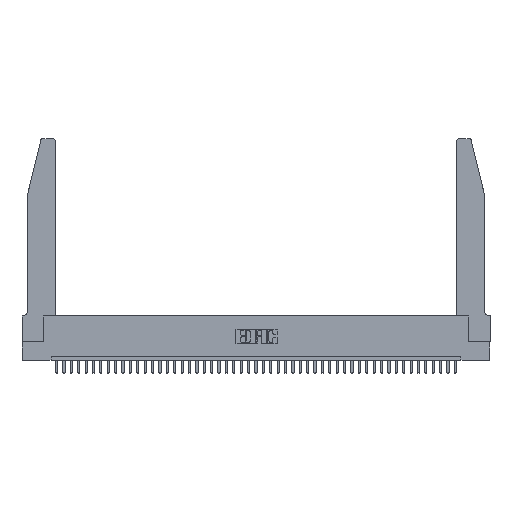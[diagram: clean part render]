
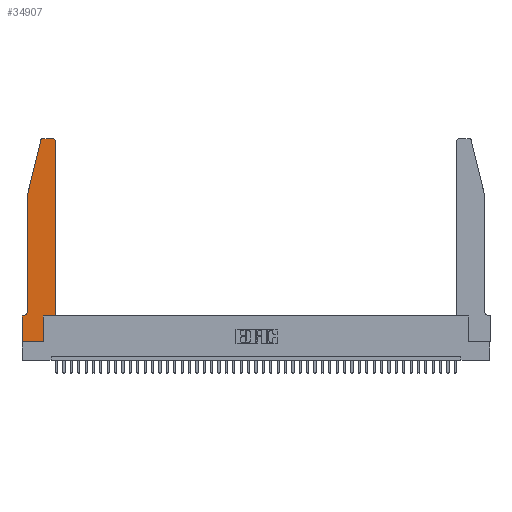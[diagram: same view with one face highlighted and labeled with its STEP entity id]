
A CAD part, top view. The second image highlights one B-rep face of the part: STEP entity #34907.
In plain terms, the highlighted planar face has unit normal (0, 0, 1).
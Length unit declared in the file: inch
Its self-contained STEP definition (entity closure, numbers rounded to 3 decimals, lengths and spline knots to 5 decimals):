
#297 = DIRECTION ( 'NONE',  ( 1., 0., 0. ) ) ;
#403 = CARTESIAN_POINT ( 'NONE',  ( 0., 0.35, 0.37 ) ) ;
#1978 = EDGE_CURVE ( 'NONE', #20768, #39292, #31162, .T. ) ;
#2014 = DIRECTION ( 'NONE',  ( -0.239, -0.971, 0. ) ) ;
#2106 = ORIENTED_EDGE ( 'NONE', *, *, #39608, .T. ) ;
#2796 = LINE ( 'NONE', #20303, #14570 ) ;
#3022 = EDGE_CURVE ( 'NONE', #9658, #12746, #7732, .T. ) ;
#3857 = EDGE_CURVE ( 'NONE', #33900, #9658, #42615, .T. ) ;
#4314 = EDGE_CURVE ( 'NONE', #7979, #17851, #2796, .T. ) ;
#4957 = CARTESIAN_POINT ( 'NONE',  ( 0.284, 2.75, 0.37 ) ) ;
#5956 = AXIS2_PLACEMENT_3D ( 'NONE', #39282, #18823, #28895 ) ;
#6140 = DIRECTION ( 'NONE',  ( 1., 0., 0. ) ) ;
#6645 = VECTOR ( 'NONE', #2014, 39.37008 ) ;
#6658 = DIRECTION ( 'NONE',  ( 0., 1., 0. ) ) ;
#6995 = CARTESIAN_POINT ( 'NONE',  ( 0.4505, 0.35, 0.37 ) ) ;
#7254 = VERTEX_POINT ( 'NONE', #19787 ) ;
#7298 = PLANE ( 'NONE',  #24226 ) ;
#7732 = LINE ( 'NONE', #34186, #6645 ) ;
#7979 = VERTEX_POINT ( 'NONE', #23984 ) ;
#8197 = ORIENTED_EDGE ( 'NONE', *, *, #4314, .T. ) ;
#9658 = VERTEX_POINT ( 'NONE', #10360 ) ;
#9827 = DIRECTION ( 'NONE',  ( 0., 0., 1. ) ) ;
#10360 = CARTESIAN_POINT ( 'NONE',  ( 0.25487, 2.72718, 0.37 ) ) ;
#10837 = CARTESIAN_POINT ( 'NONE',  ( 0.0755, 2., 0.37 ) ) ;
#10908 = DIRECTION ( 'NONE',  ( 1., 0., 0. ) ) ;
#11545 = CARTESIAN_POINT ( 'NONE',  ( 0.2865, 0.35, 0.37 ) ) ;
#11945 = CARTESIAN_POINT ( 'NONE',  ( 0.4505, 0.35, 0.37 ) ) ;
#12109 = DIRECTION ( 'NONE',  ( 0., 1., 0. ) ) ;
#12197 = CARTESIAN_POINT ( 'NONE',  ( 0., 0., 0.37 ) ) ;
#12203 = VECTOR ( 'NONE', #297, 39.37008 ) ;
#12720 = ORIENTED_EDGE ( 'NONE', *, *, #3857, .T. ) ;
#12746 = VERTEX_POINT ( 'NONE', #10837 ) ;
#12932 = LINE ( 'NONE', #32423, #36045 ) ;
#13054 = DIRECTION ( 'NONE',  ( 0., 0., 1. ) ) ;
#13738 = VERTEX_POINT ( 'NONE', #14150 ) ;
#13890 = CARTESIAN_POINT ( 'NONE',  ( 0.4505, 2.72, 0.37 ) ) ;
#14033 = CIRCLE ( 'NONE', #5956, 0.07 ) ;
#14150 = CARTESIAN_POINT ( 'NONE',  ( 0.4205, 2.75, 0.37 ) ) ;
#14570 = VECTOR ( 'NONE', #6658, 39.37008 ) ;
#14642 = EDGE_LOOP ( 'NONE', ( #20330, #12720, #42445, #37048, #2106, #18163, #32972, #26122, #8197, #28283, #30960, #26361 ) ) ;
#14830 = DIRECTION ( 'NONE',  ( -1., 0., 0. ) ) ;
#15657 = DIRECTION ( 'NONE',  ( 0., -1., 0. ) ) ;
#16758 = EDGE_CURVE ( 'NONE', #17851, #20768, #31568, .T. ) ;
#17401 = LINE ( 'NONE', #12197, #41086 ) ;
#17851 = VERTEX_POINT ( 'NONE', #11545 ) ;
#18163 = ORIENTED_EDGE ( 'NONE', *, *, #20363, .T. ) ;
#18823 = DIRECTION ( 'NONE',  ( 0., 0., -1. ) ) ;
#19651 = VECTOR ( 'NONE', #28076, 39.37008 ) ;
#19787 = CARTESIAN_POINT ( 'NONE',  ( 0., 0.35, 0.37 ) ) ;
#20303 = CARTESIAN_POINT ( 'NONE',  ( 0.2865, 0.35, 0.37 ) ) ;
#20330 = ORIENTED_EDGE ( 'NONE', *, *, #34565, .T. ) ;
#20346 = AXIS2_PLACEMENT_3D ( 'NONE', #30419, #9827, #36890 ) ;
#20363 = EDGE_CURVE ( 'NONE', #42018, #7254, #39088, .T. ) ;
#20561 = CARTESIAN_POINT ( 'NONE',  ( 0., 0., 0.37 ) ) ;
#20768 = VERTEX_POINT ( 'NONE', #6995 ) ;
#20901 = VECTOR ( 'NONE', #12109, 39.37008 ) ;
#21825 = VECTOR ( 'NONE', #32919, 39.37008 ) ;
#22488 = CARTESIAN_POINT ( 'NONE',  ( 0.0755, 0.35, 0.37 ) ) ;
#23387 = DIRECTION ( 'NONE',  ( 0., -1., 0. ) ) ;
#23984 = CARTESIAN_POINT ( 'NONE',  ( 0.2865, 0., 0.37 ) ) ;
#24226 = AXIS2_PLACEMENT_3D ( 'NONE', #403, #34671, #10908 ) ;
#24660 = FACE_OUTER_BOUND ( 'NONE', #14642, .T. ) ;
#26122 = ORIENTED_EDGE ( 'NONE', *, *, #43389, .T. ) ;
#26350 = EDGE_CURVE ( 'NONE', #12746, #31910, #37922, .T. ) ;
#26361 = ORIENTED_EDGE ( 'NONE', *, *, #39867, .T. ) ;
#26746 = AXIS2_PLACEMENT_3D ( 'NONE', #33659, #13054, #6140 ) ;
#27001 = CARTESIAN_POINT ( 'NONE',  ( 0.0055, 0.35, 0.37 ) ) ;
#27049 = CARTESIAN_POINT ( 'NONE',  ( 0.0755, 0.42, 0.37 ) ) ;
#27430 = CIRCLE ( 'NONE', #20346, 0.03 ) ;
#27991 = EDGE_CURVE ( 'NONE', #7254, #29210, #17401, .T. ) ;
#28076 = DIRECTION ( 'NONE',  ( 1., 0., 0. ) ) ;
#28283 = ORIENTED_EDGE ( 'NONE', *, *, #16758, .T. ) ;
#28895 = DIRECTION ( 'NONE',  ( -1., 0., 0. ) ) ;
#29210 = VERTEX_POINT ( 'NONE', #39020 ) ;
#30051 = CARTESIAN_POINT ( 'NONE',  ( 0.0755, 2., 0.37 ) ) ;
#30419 = CARTESIAN_POINT ( 'NONE',  ( 0.4205, 2.72, 0.37 ) ) ;
#30960 = ORIENTED_EDGE ( 'NONE', *, *, #1978, .T. ) ;
#31162 = LINE ( 'NONE', #11945, #20901 ) ;
#31568 = LINE ( 'NONE', #41604, #12203 ) ;
#31910 = VERTEX_POINT ( 'NONE', #27049 ) ;
#32423 = CARTESIAN_POINT ( 'NONE',  ( 0.2605, 2.75, 0.37 ) ) ;
#32919 = DIRECTION ( 'NONE',  ( -1., 0., 0. ) ) ;
#32972 = ORIENTED_EDGE ( 'NONE', *, *, #27991, .T. ) ;
#33659 = CARTESIAN_POINT ( 'NONE',  ( 0.284, 2.72, 0.37 ) ) ;
#33900 = VERTEX_POINT ( 'NONE', #4957 ) ;
#34186 = CARTESIAN_POINT ( 'NONE',  ( 0.0755, 2., 0.37 ) ) ;
#34565 = EDGE_CURVE ( 'NONE', #13738, #33900, #12932, .T. ) ;
#34671 = DIRECTION ( 'NONE',  ( 0., 0., 1. ) ) ;
#34907 = ADVANCED_FACE ( 'NONE', ( #24660 ), #7298, .T. ) ;
#36045 = VECTOR ( 'NONE', #14830, 39.37008 ) ;
#36890 = DIRECTION ( 'NONE',  ( 1., 0., 0. ) ) ;
#37048 = ORIENTED_EDGE ( 'NONE', *, *, #26350, .T. ) ;
#37922 = LINE ( 'NONE', #30051, #40641 ) ;
#39020 = CARTESIAN_POINT ( 'NONE',  ( 0., 0., 0.37 ) ) ;
#39088 = LINE ( 'NONE', #22488, #21825 ) ;
#39282 = CARTESIAN_POINT ( 'NONE',  ( 0.0055, 0.42, 0.37 ) ) ;
#39292 = VERTEX_POINT ( 'NONE', #13890 ) ;
#39608 = EDGE_CURVE ( 'NONE', #31910, #42018, #14033, .T. ) ;
#39867 = EDGE_CURVE ( 'NONE', #39292, #13738, #27430, .T. ) ;
#40117 = LINE ( 'NONE', #20561, #19651 ) ;
#40641 = VECTOR ( 'NONE', #23387, 39.37008 ) ;
#41086 = VECTOR ( 'NONE', #15657, 39.37008 ) ;
#41604 = CARTESIAN_POINT ( 'NONE',  ( 0.4505, 0.35, 0.37 ) ) ;
#42018 = VERTEX_POINT ( 'NONE', #27001 ) ;
#42445 = ORIENTED_EDGE ( 'NONE', *, *, #3022, .T. ) ;
#42615 = CIRCLE ( 'NONE', #26746, 0.03 ) ;
#43389 = EDGE_CURVE ( 'NONE', #29210, #7979, #40117, .T. ) ;
